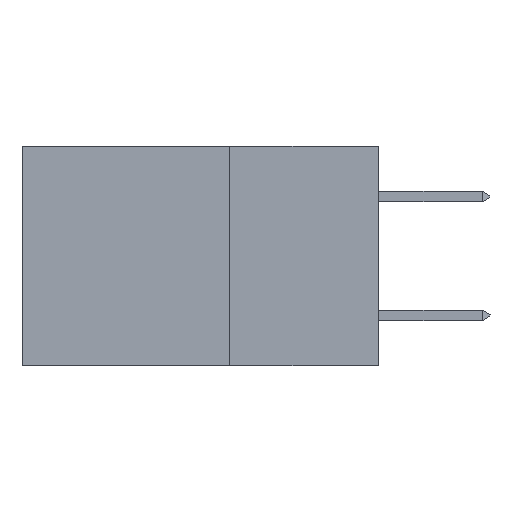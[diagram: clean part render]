
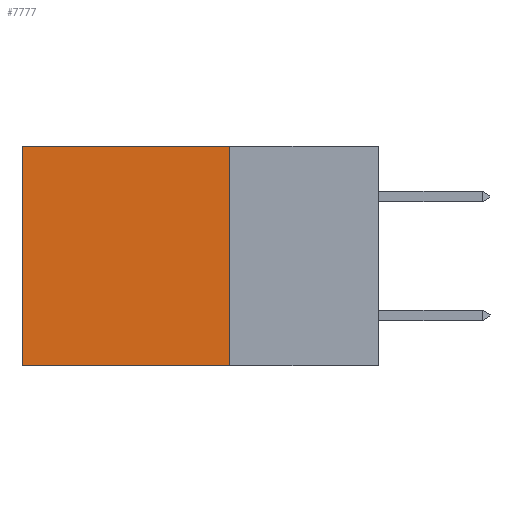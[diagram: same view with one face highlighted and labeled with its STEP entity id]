
A CAD part, left-side view. The second image highlights one B-rep face of the part: STEP entity #7777.
In plain terms, the highlighted planar face has unit normal (-1, 0, 0).
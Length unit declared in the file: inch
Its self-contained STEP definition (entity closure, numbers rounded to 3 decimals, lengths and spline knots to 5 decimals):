
#306 = DIRECTION ( 'NONE',  ( 0., 0., -1. ) ) ;
#2384 = ORIENTED_EDGE ( 'NONE', *, *, #11775, .T. ) ;
#2945 = DIRECTION ( 'NONE',  ( 0., 0., -1. ) ) ;
#3369 = EDGE_CURVE ( 'NONE', #11691, #15684, #25360, .T. ) ;
#4015 = VECTOR ( 'NONE', #20891, 39.37008 ) ;
#4041 = LINE ( 'NONE', #6567, #4015 ) ;
#4853 = DIRECTION ( 'NONE',  ( 0., 0., -1. ) ) ;
#6277 = EDGE_CURVE ( 'NONE', #15684, #15326, #19070, .T. ) ;
#6567 = CARTESIAN_POINT ( 'NONE',  ( 0.298, 0.25, 0. ) ) ;
#7777 = ADVANCED_FACE ( 'NONE', ( #10403 ), #15074, .F. ) ;
#7957 = ORIENTED_EDGE ( 'NONE', *, *, #19239, .T. ) ;
#8186 = CARTESIAN_POINT ( 'NONE',  ( 0.298, 0.25, -0.37 ) ) ;
#8670 = VECTOR ( 'NONE', #306, 39.37008 ) ;
#10403 = FACE_OUTER_BOUND ( 'NONE', #23899, .T. ) ;
#11225 = DIRECTION ( 'NONE',  ( 1., 0., 0. ) ) ;
#11691 = VERTEX_POINT ( 'NONE', #18389 ) ;
#11775 = EDGE_CURVE ( 'NONE', #11691, #22163, #4041, .T. ) ;
#12588 = CARTESIAN_POINT ( 'NONE',  ( 0.298, 0.25, -0.37 ) ) ;
#12948 = VECTOR ( 'NONE', #2945, 39.37008 ) ;
#15074 = PLANE ( 'NONE',  #23655 ) ;
#15326 = VERTEX_POINT ( 'NONE', #25836 ) ;
#15684 = VERTEX_POINT ( 'NONE', #12588 ) ;
#15842 = CARTESIAN_POINT ( 'NONE',  ( 0.298, 0.6, 0. ) ) ;
#15996 = CARTESIAN_POINT ( 'NONE',  ( 0.298, 0.6, 0. ) ) ;
#18389 = CARTESIAN_POINT ( 'NONE',  ( 0.298, 0.25, 0. ) ) ;
#19070 = LINE ( 'NONE', #8186, #19750 ) ;
#19239 = EDGE_CURVE ( 'NONE', #22163, #15326, #21124, .T. ) ;
#19542 = CARTESIAN_POINT ( 'NONE',  ( 0.298, 0.25, 0. ) ) ;
#19750 = VECTOR ( 'NONE', #23434, 39.37008 ) ;
#20348 = ORIENTED_EDGE ( 'NONE', *, *, #6277, .F. ) ;
#20891 = DIRECTION ( 'NONE',  ( 0., 1., 0. ) ) ;
#21124 = LINE ( 'NONE', #15996, #12948 ) ;
#22163 = VERTEX_POINT ( 'NONE', #15842 ) ;
#23434 = DIRECTION ( 'NONE',  ( 0., 1., 0. ) ) ;
#23655 = AXIS2_PLACEMENT_3D ( 'NONE', #19542, #11225, #4853 ) ;
#23899 = EDGE_LOOP ( 'NONE', ( #7957, #20348, #27478, #2384 ) ) ;
#25360 = LINE ( 'NONE', #26420, #8670 ) ;
#25836 = CARTESIAN_POINT ( 'NONE',  ( 0.298, 0.6, -0.37 ) ) ;
#26420 = CARTESIAN_POINT ( 'NONE',  ( 0.298, 0.25, 0. ) ) ;
#27478 = ORIENTED_EDGE ( 'NONE', *, *, #3369, .F. ) ;
